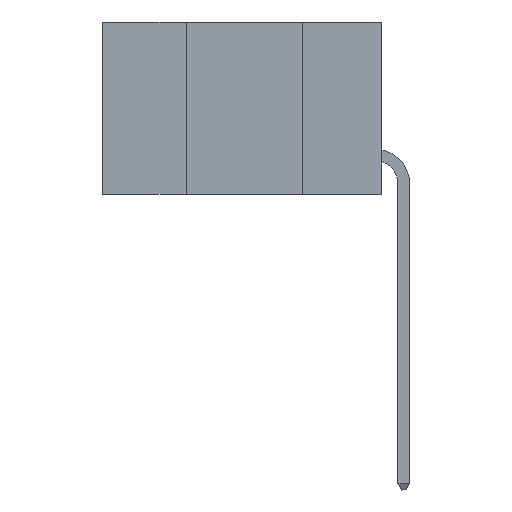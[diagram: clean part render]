
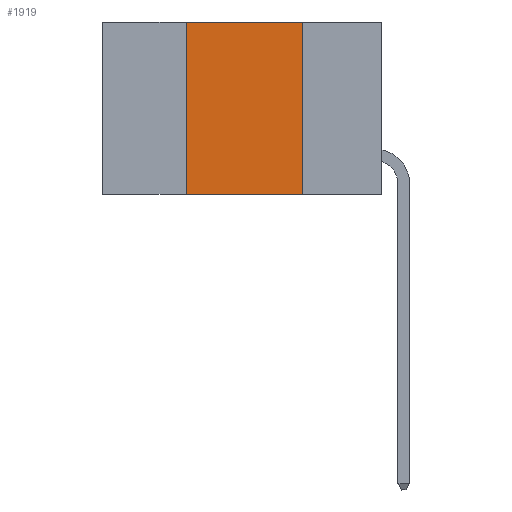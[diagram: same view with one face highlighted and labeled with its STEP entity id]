
A CAD part, left-side view. The second image highlights one B-rep face of the part: STEP entity #1919.
In plain terms, the highlighted planar face has unit normal (-1, 0, 0).
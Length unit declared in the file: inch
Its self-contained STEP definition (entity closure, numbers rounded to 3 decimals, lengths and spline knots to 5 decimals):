
#45 = ORIENTED_EDGE ( 'NONE', *, *, #15222, .F. ) ;
#1530 = ORIENTED_EDGE ( 'NONE', *, *, #5284, .T. ) ;
#1576 = CARTESIAN_POINT ( 'NONE',  ( 0., 0.42, 0. ) ) ;
#1919 = ADVANCED_FACE ( 'NONE', ( #14062 ), #13756, .F. ) ;
#2802 = CARTESIAN_POINT ( 'NONE',  ( 0., 0.6, 0. ) ) ;
#2941 = VERTEX_POINT ( 'NONE', #16154 ) ;
#4200 = VERTEX_POINT ( 'NONE', #14411 ) ;
#4448 = LINE ( 'NONE', #15687, #15501 ) ;
#4489 = VERTEX_POINT ( 'NONE', #5719 ) ;
#4941 = DIRECTION ( 'NONE',  ( 1., 0., 0. ) ) ;
#5284 = EDGE_CURVE ( 'NONE', #4200, #15040, #14347, .T. ) ;
#5460 = AXIS2_PLACEMENT_3D ( 'NONE', #7422, #4941, #8801 ) ;
#5719 = CARTESIAN_POINT ( 'NONE',  ( 0., 0.17, 0. ) ) ;
#5872 = DIRECTION ( 'NONE',  ( 0., -1., 0. ) ) ;
#6539 = DIRECTION ( 'NONE',  ( 0., -1., 0. ) ) ;
#6594 = VECTOR ( 'NONE', #6539, 39.37008 ) ;
#7422 = CARTESIAN_POINT ( 'NONE',  ( 0., 0.6, 0. ) ) ;
#7736 = EDGE_CURVE ( 'NONE', #4489, #15040, #4448, .T. ) ;
#8269 = CARTESIAN_POINT ( 'NONE',  ( 0., 0.6, -0.37 ) ) ;
#8473 = CARTESIAN_POINT ( 'NONE',  ( 0., 0.17, -0.37 ) ) ;
#8715 = ORIENTED_EDGE ( 'NONE', *, *, #7736, .F. ) ;
#8801 = DIRECTION ( 'NONE',  ( 0., 0., -1. ) ) ;
#9935 = LINE ( 'NONE', #2802, #6594 ) ;
#10598 = LINE ( 'NONE', #1576, #15571 ) ;
#11012 = EDGE_CURVE ( 'NONE', #2941, #4489, #9935, .T. ) ;
#11278 = ORIENTED_EDGE ( 'NONE', *, *, #11012, .F. ) ;
#11398 = EDGE_LOOP ( 'NONE', ( #8715, #11278, #45, #1530 ) ) ;
#11667 = DIRECTION ( 'NONE',  ( 0., 0., 1. ) ) ;
#13016 = DIRECTION ( 'NONE',  ( 0., 0., -1. ) ) ;
#13756 = PLANE ( 'NONE',  #5460 ) ;
#14062 = FACE_OUTER_BOUND ( 'NONE', #11398, .T. ) ;
#14347 = LINE ( 'NONE', #8269, #15954 ) ;
#14411 = CARTESIAN_POINT ( 'NONE',  ( 0., 0.42, -0.37 ) ) ;
#15040 = VERTEX_POINT ( 'NONE', #8473 ) ;
#15222 = EDGE_CURVE ( 'NONE', #4200, #2941, #10598, .T. ) ;
#15501 = VECTOR ( 'NONE', #13016, 39.37008 ) ;
#15571 = VECTOR ( 'NONE', #11667, 39.37008 ) ;
#15687 = CARTESIAN_POINT ( 'NONE',  ( 0., 0.17, 0. ) ) ;
#15954 = VECTOR ( 'NONE', #5872, 39.37008 ) ;
#16154 = CARTESIAN_POINT ( 'NONE',  ( 0., 0.42, 0. ) ) ;
